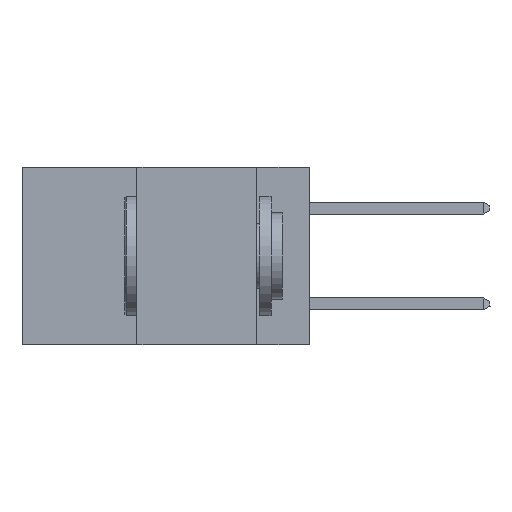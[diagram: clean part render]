
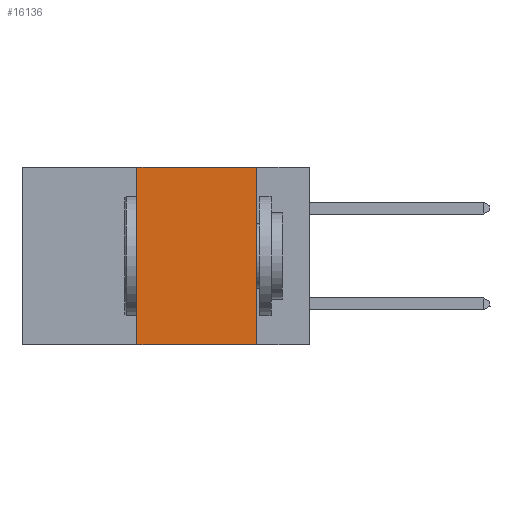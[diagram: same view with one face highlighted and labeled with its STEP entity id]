
A CAD part, left-side view. The second image highlights one B-rep face of the part: STEP entity #16136.
In plain terms, the highlighted planar face has unit normal (-1, 0, 0).
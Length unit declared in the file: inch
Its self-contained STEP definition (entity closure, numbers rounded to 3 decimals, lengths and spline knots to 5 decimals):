
#561 = CARTESIAN_POINT ( 'NONE',  ( 0., 0.11, -0.37 ) ) ;
#950 = VERTEX_POINT ( 'NONE', #4621 ) ;
#1005 = DIRECTION ( 'NONE',  ( 0., 0., -1. ) ) ;
#1719 = CARTESIAN_POINT ( 'NONE',  ( 0., 0.6, -0.37 ) ) ;
#1791 = VECTOR ( 'NONE', #15084, 39.37008 ) ;
#1982 = ORIENTED_EDGE ( 'NONE', *, *, #2567, .T. ) ;
#2150 = VECTOR ( 'NONE', #7605, 39.37008 ) ;
#2567 = EDGE_CURVE ( 'NONE', #9712, #3260, #6975, .T. ) ;
#2748 = VECTOR ( 'NONE', #5562, 39.37008 ) ;
#2843 = ORIENTED_EDGE ( 'NONE', *, *, #6066, .F. ) ;
#3203 = EDGE_CURVE ( 'NONE', #950, #3260, #14209, .T. ) ;
#3260 = VERTEX_POINT ( 'NONE', #561 ) ;
#3987 = VERTEX_POINT ( 'NONE', #14382 ) ;
#4339 = CARTESIAN_POINT ( 'NONE',  ( 0., 0.11, 0. ) ) ;
#4621 = CARTESIAN_POINT ( 'NONE',  ( 0., 0.11, 0. ) ) ;
#4771 = CARTESIAN_POINT ( 'NONE',  ( 0., 0.36, 0. ) ) ;
#5562 = DIRECTION ( 'NONE',  ( 0., -1., 0. ) ) ;
#6066 = EDGE_CURVE ( 'NONE', #9712, #3987, #13948, .T. ) ;
#6167 = DIRECTION ( 'NONE',  ( 1., 0., 0. ) ) ;
#6515 = ORIENTED_EDGE ( 'NONE', *, *, #15484, .F. ) ;
#6975 = LINE ( 'NONE', #1719, #2748 ) ;
#7605 = DIRECTION ( 'NONE',  ( 0., 0., 1. ) ) ;
#8685 = FACE_OUTER_BOUND ( 'NONE', #16772, .T. ) ;
#8730 = VECTOR ( 'NONE', #14665, 39.37008 ) ;
#9712 = VERTEX_POINT ( 'NONE', #15285 ) ;
#10034 = CARTESIAN_POINT ( 'NONE',  ( 0., 0.6, 0. ) ) ;
#10411 = AXIS2_PLACEMENT_3D ( 'NONE', #16635, #6167, #1005 ) ;
#12937 = PLANE ( 'NONE',  #10411 ) ;
#13449 = ORIENTED_EDGE ( 'NONE', *, *, #3203, .F. ) ;
#13948 = LINE ( 'NONE', #4771, #2150 ) ;
#14013 = LINE ( 'NONE', #10034, #1791 ) ;
#14209 = LINE ( 'NONE', #4339, #8730 ) ;
#14382 = CARTESIAN_POINT ( 'NONE',  ( 0., 0.36, 0. ) ) ;
#14665 = DIRECTION ( 'NONE',  ( 0., 0., -1. ) ) ;
#15084 = DIRECTION ( 'NONE',  ( 0., -1., 0. ) ) ;
#15285 = CARTESIAN_POINT ( 'NONE',  ( 0., 0.36, -0.37 ) ) ;
#15484 = EDGE_CURVE ( 'NONE', #3987, #950, #14013, .T. ) ;
#16136 = ADVANCED_FACE ( 'NONE', ( #8685 ), #12937, .F. ) ;
#16635 = CARTESIAN_POINT ( 'NONE',  ( 0., 0.6, 0. ) ) ;
#16772 = EDGE_LOOP ( 'NONE', ( #13449, #6515, #2843, #1982 ) ) ;
